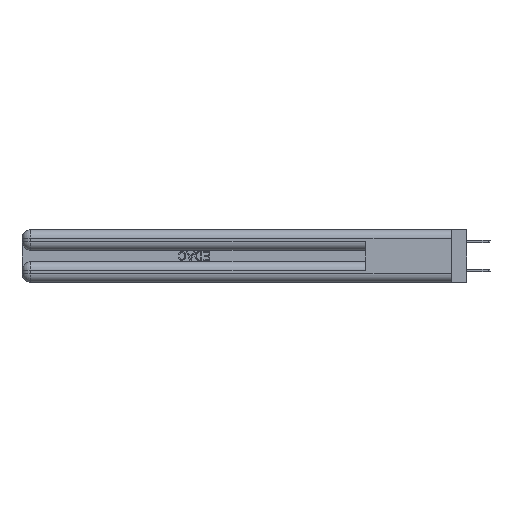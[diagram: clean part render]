
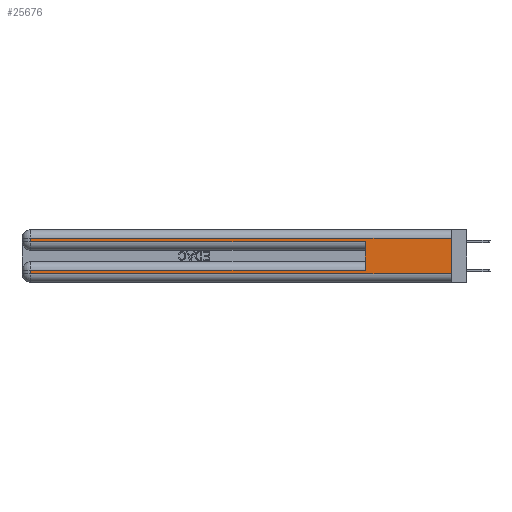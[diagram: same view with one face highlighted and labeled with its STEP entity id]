
A CAD part, left-side view. The second image highlights one B-rep face of the part: STEP entity #25676.
In plain terms, the highlighted planar face has unit normal (-1, 0, 0).
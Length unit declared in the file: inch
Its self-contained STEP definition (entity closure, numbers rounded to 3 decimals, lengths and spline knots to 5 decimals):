
#805 = EDGE_CURVE ( 'NONE', #15269, #3546, #4627, .T. ) ;
#1437 = VERTEX_POINT ( 'NONE', #16929 ) ;
#2191 = LINE ( 'NONE', #23446, #21874 ) ;
#2426 = EDGE_LOOP ( 'NONE', ( #12254, #3394, #40978, #3339, #12758, #7736, #43347, #3835 ) ) ;
#3339 = ORIENTED_EDGE ( 'NONE', *, *, #33125, .T. ) ;
#3394 = ORIENTED_EDGE ( 'NONE', *, *, #27751, .T. ) ;
#3546 = VERTEX_POINT ( 'NONE', #32632 ) ;
#3635 = EDGE_CURVE ( 'NONE', #1437, #5974, #45522, .T. ) ;
#3835 = ORIENTED_EDGE ( 'NONE', *, *, #3635, .T. ) ;
#3939 = VECTOR ( 'NONE', #15379, 39.37008 ) ;
#4153 = DIRECTION ( 'NONE',  ( 0., 1., 0. ) ) ;
#4627 = LINE ( 'NONE', #35644, #24257 ) ;
#4705 = DIRECTION ( 'NONE',  ( 0., 0., -1. ) ) ;
#5974 = VERTEX_POINT ( 'NONE', #13895 ) ;
#7736 = ORIENTED_EDGE ( 'NONE', *, *, #36939, .T. ) ;
#7928 = CARTESIAN_POINT ( 'NONE',  ( 0., 2.94, 0.31 ) ) ;
#11008 = DIRECTION ( 'NONE',  ( 0., -1., 0. ) ) ;
#11672 = CARTESIAN_POINT ( 'NONE',  ( 0., 0., 0.37 ) ) ;
#11892 = CARTESIAN_POINT ( 'NONE',  ( 0., 0., 0.31 ) ) ;
#12254 = ORIENTED_EDGE ( 'NONE', *, *, #24923, .F. ) ;
#12380 = DIRECTION ( 'NONE',  ( 0., -1., 0. ) ) ;
#12758 = ORIENTED_EDGE ( 'NONE', *, *, #805, .F. ) ;
#13763 = DIRECTION ( 'NONE',  ( 0., 0., 1. ) ) ;
#13895 = CARTESIAN_POINT ( 'NONE',  ( 0., 0., 0.06 ) ) ;
#14974 = LINE ( 'NONE', #11672, #3939 ) ;
#15269 = VERTEX_POINT ( 'NONE', #37022 ) ;
#15379 = DIRECTION ( 'NONE',  ( 0., 0., -1. ) ) ;
#15959 = CARTESIAN_POINT ( 'NONE',  ( 0., 2.94, 0.085 ) ) ;
#16285 = DIRECTION ( 'NONE',  ( 1., 0., 0. ) ) ;
#16929 = CARTESIAN_POINT ( 'NONE',  ( 0., 2.94, 0.06 ) ) ;
#18071 = VERTEX_POINT ( 'NONE', #7928 ) ;
#19995 = DIRECTION ( 'NONE',  ( 0., 0., -1. ) ) ;
#20952 = VERTEX_POINT ( 'NONE', #25963 ) ;
#21673 = LINE ( 'NONE', #11892, #30239 ) ;
#21874 = VECTOR ( 'NONE', #12380, 39.37008 ) ;
#21892 = LINE ( 'NONE', #23103, #23018 ) ;
#23018 = VECTOR ( 'NONE', #4705, 39.37008 ) ;
#23103 = CARTESIAN_POINT ( 'NONE',  ( 0., 2.94, 0.37 ) ) ;
#23446 = CARTESIAN_POINT ( 'NONE',  ( 0., 0., 0.285 ) ) ;
#23715 = VERTEX_POINT ( 'NONE', #15959 ) ;
#24257 = VECTOR ( 'NONE', #13763, 39.37008 ) ;
#24635 = VECTOR ( 'NONE', #4153, 39.37008 ) ;
#24923 = EDGE_CURVE ( 'NONE', #28636, #5974, #14974, .T. ) ;
#25676 = ADVANCED_FACE ( 'NONE', ( #32157 ), #27172, .F. ) ;
#25963 = CARTESIAN_POINT ( 'NONE',  ( 0., 2.94, 0.285 ) ) ;
#26213 = VECTOR ( 'NONE', #11008, 39.37008 ) ;
#26228 = CARTESIAN_POINT ( 'NONE',  ( 0., 0., 0.085 ) ) ;
#26644 = DIRECTION ( 'NONE',  ( 0., 1., 0. ) ) ;
#27172 = PLANE ( 'NONE',  #40238 ) ;
#27343 = CARTESIAN_POINT ( 'NONE',  ( 0., 2.94, 0.37 ) ) ;
#27751 = EDGE_CURVE ( 'NONE', #28636, #18071, #21673, .T. ) ;
#27756 = VECTOR ( 'NONE', #19995, 39.37008 ) ;
#28636 = VERTEX_POINT ( 'NONE', #32160 ) ;
#30239 = VECTOR ( 'NONE', #26644, 39.37008 ) ;
#30915 = LINE ( 'NONE', #26228, #24635 ) ;
#32157 = FACE_OUTER_BOUND ( 'NONE', #2426, .T. ) ;
#32160 = CARTESIAN_POINT ( 'NONE',  ( 0., 0., 0.31 ) ) ;
#32632 = CARTESIAN_POINT ( 'NONE',  ( 0., 0.6, 0.285 ) ) ;
#33125 = EDGE_CURVE ( 'NONE', #20952, #3546, #2191, .T. ) ;
#35644 = CARTESIAN_POINT ( 'NONE',  ( 0., 0.6, 0.145 ) ) ;
#35849 = EDGE_CURVE ( 'NONE', #23715, #1437, #21892, .T. ) ;
#36939 = EDGE_CURVE ( 'NONE', #15269, #23715, #30915, .T. ) ;
#37022 = CARTESIAN_POINT ( 'NONE',  ( 0., 0.6, 0.085 ) ) ;
#37837 = CARTESIAN_POINT ( 'NONE',  ( 0., 0., 0.06 ) ) ;
#40238 = AXIS2_PLACEMENT_3D ( 'NONE', #45091, #16285, #41791 ) ;
#40633 = EDGE_CURVE ( 'NONE', #18071, #20952, #47066, .T. ) ;
#40978 = ORIENTED_EDGE ( 'NONE', *, *, #40633, .T. ) ;
#41791 = DIRECTION ( 'NONE',  ( 0., 0., -1. ) ) ;
#43347 = ORIENTED_EDGE ( 'NONE', *, *, #35849, .T. ) ;
#45091 = CARTESIAN_POINT ( 'NONE',  ( 0., 0., 0.37 ) ) ;
#45522 = LINE ( 'NONE', #37837, #26213 ) ;
#47066 = LINE ( 'NONE', #27343, #27756 ) ;
